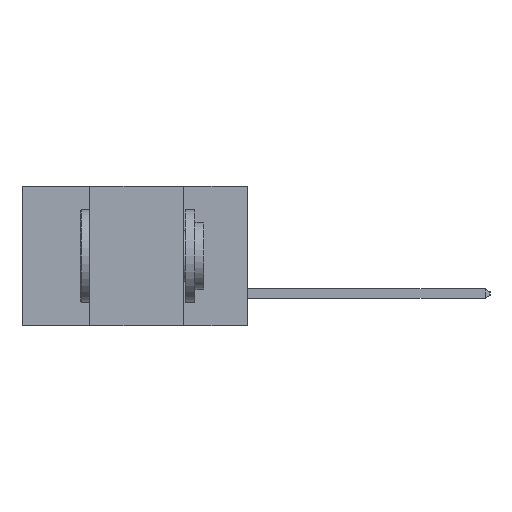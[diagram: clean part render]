
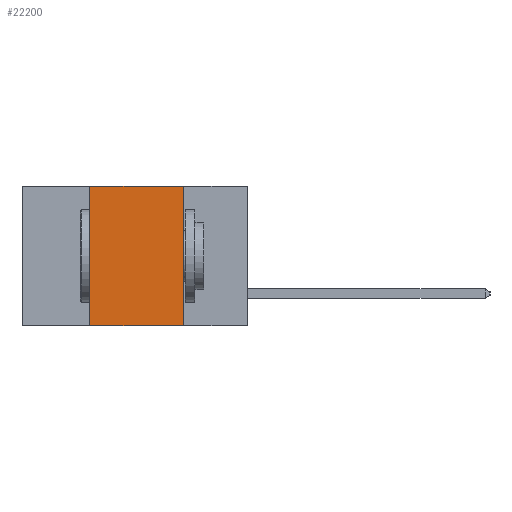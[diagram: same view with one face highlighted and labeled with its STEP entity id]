
A CAD part, left-side view. The second image highlights one B-rep face of the part: STEP entity #22200.
In plain terms, the highlighted planar face has unit normal (-1, 0, 0).
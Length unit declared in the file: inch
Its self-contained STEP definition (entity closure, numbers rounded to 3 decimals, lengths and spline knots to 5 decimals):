
#39 = ORIENTED_EDGE ( 'NONE', *, *, #20447, .F. ) ;
#238 = CARTESIAN_POINT ( 'NONE',  ( 0., 0.17, -0.37 ) ) ;
#912 = VECTOR ( 'NONE', #22156, 39.37008 ) ;
#1229 = DIRECTION ( 'NONE',  ( 0., 0., -1. ) ) ;
#2305 = CARTESIAN_POINT ( 'NONE',  ( 0., 0.42, 0. ) ) ;
#2328 = DIRECTION ( 'NONE',  ( 0., 0., -1. ) ) ;
#3974 = LINE ( 'NONE', #238, #19749 ) ;
#5334 = CARTESIAN_POINT ( 'NONE',  ( 0., 0.42, -0.37 ) ) ;
#5775 = AXIS2_PLACEMENT_3D ( 'NONE', #21707, #13612, #1229 ) ;
#5889 = ORIENTED_EDGE ( 'NONE', *, *, #25804, .F. ) ;
#6694 = ORIENTED_EDGE ( 'NONE', *, *, #9843, .F. ) ;
#6715 = EDGE_CURVE ( 'NONE', #8187, #13741, #16748, .T. ) ;
#8187 = VERTEX_POINT ( 'NONE', #5334 ) ;
#8200 = CARTESIAN_POINT ( 'NONE',  ( 0., 0.42, -0.37 ) ) ;
#9658 = LINE ( 'NONE', #8200, #25206 ) ;
#9843 = EDGE_CURVE ( 'NONE', #17292, #13741, #3974, .T. ) ;
#10275 = DIRECTION ( 'NONE',  ( 0., 0., 1. ) ) ;
#11535 = PLANE ( 'NONE',  #5775 ) ;
#11923 = LINE ( 'NONE', #20140, #912 ) ;
#13612 = DIRECTION ( 'NONE',  ( 1., 0., 0. ) ) ;
#13741 = VERTEX_POINT ( 'NONE', #25830 ) ;
#16116 = VECTOR ( 'NONE', #20255, 39.37008 ) ;
#16538 = ORIENTED_EDGE ( 'NONE', *, *, #6715, .T. ) ;
#16748 = LINE ( 'NONE', #20027, #16116 ) ;
#17292 = VERTEX_POINT ( 'NONE', #18278 ) ;
#18278 = CARTESIAN_POINT ( 'NONE',  ( 0., 0.17, 0. ) ) ;
#19749 = VECTOR ( 'NONE', #2328, 39.37008 ) ;
#20027 = CARTESIAN_POINT ( 'NONE',  ( 0., 0.6, -0.37 ) ) ;
#20140 = CARTESIAN_POINT ( 'NONE',  ( 0., 0.6, 0. ) ) ;
#20255 = DIRECTION ( 'NONE',  ( 0., -1., 0. ) ) ;
#20447 = EDGE_CURVE ( 'NONE', #8187, #26064, #9658, .T. ) ;
#21707 = CARTESIAN_POINT ( 'NONE',  ( 0., 0.6, 0. ) ) ;
#22156 = DIRECTION ( 'NONE',  ( 0., -1., 0. ) ) ;
#22200 = ADVANCED_FACE ( 'NONE', ( #24200 ), #11535, .F. ) ;
#24200 = FACE_OUTER_BOUND ( 'NONE', #25939, .T. ) ;
#25206 = VECTOR ( 'NONE', #10275, 39.37008 ) ;
#25804 = EDGE_CURVE ( 'NONE', #26064, #17292, #11923, .T. ) ;
#25830 = CARTESIAN_POINT ( 'NONE',  ( 0., 0.17, -0.37 ) ) ;
#25939 = EDGE_LOOP ( 'NONE', ( #6694, #5889, #39, #16538 ) ) ;
#26064 = VERTEX_POINT ( 'NONE', #2305 ) ;
